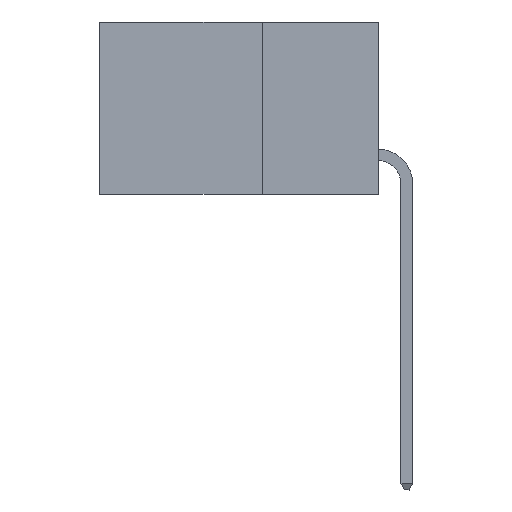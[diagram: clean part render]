
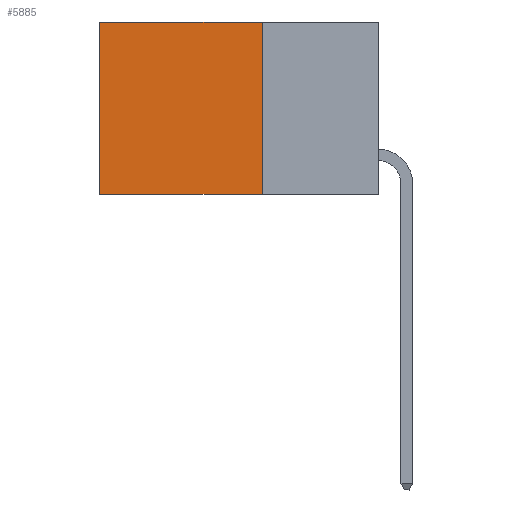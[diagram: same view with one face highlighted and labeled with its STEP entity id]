
A CAD part, left-side view. The second image highlights one B-rep face of the part: STEP entity #5885.
In plain terms, the highlighted planar face has unit normal (-1, 0, 0).
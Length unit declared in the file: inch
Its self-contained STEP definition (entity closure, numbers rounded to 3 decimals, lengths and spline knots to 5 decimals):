
#154 = EDGE_CURVE ( 'NONE', #14448, #2930, #10044, .T. ) ;
#266 = PLANE ( 'NONE',  #12601 ) ;
#954 = ORIENTED_EDGE ( 'NONE', *, *, #2855, .T. ) ;
#955 = CARTESIAN_POINT ( 'NONE',  ( 0.2615, 0.6, -0.37 ) ) ;
#1725 = ORIENTED_EDGE ( 'NONE', *, *, #154, .F. ) ;
#2405 = ORIENTED_EDGE ( 'NONE', *, *, #7330, .T. ) ;
#2855 = EDGE_CURVE ( 'NONE', #3892, #14859, #12479, .T. ) ;
#2923 = LINE ( 'NONE', #6515, #12404 ) ;
#2930 = VERTEX_POINT ( 'NONE', #11233 ) ;
#3892 = VERTEX_POINT ( 'NONE', #11964 ) ;
#5016 = DIRECTION ( 'NONE',  ( 0., 0., -1. ) ) ;
#5317 = CARTESIAN_POINT ( 'NONE',  ( 0.2615, 0.25, 0. ) ) ;
#5709 = DIRECTION ( 'NONE',  ( 0., 0., -1. ) ) ;
#5885 = ADVANCED_FACE ( 'NONE', ( #6194 ), #266, .F. ) ;
#6194 = FACE_OUTER_BOUND ( 'NONE', #13691, .T. ) ;
#6474 = CARTESIAN_POINT ( 'NONE',  ( 0.2615, 0.25, -0.37 ) ) ;
#6515 = CARTESIAN_POINT ( 'NONE',  ( 0.2615, 0.25, -0.37 ) ) ;
#7194 = CARTESIAN_POINT ( 'NONE',  ( 0.2615, 0.25, -0.37 ) ) ;
#7330 = EDGE_CURVE ( 'NONE', #14859, #2930, #11626, .T. ) ;
#8053 = EDGE_CURVE ( 'NONE', #3892, #14448, #2923, .T. ) ;
#8152 = VECTOR ( 'NONE', #5709, 39.37008 ) ;
#8535 = VECTOR ( 'NONE', #9901, 39.37008 ) ;
#9164 = DIRECTION ( 'NONE',  ( 0., 0., -1. ) ) ;
#9699 = CARTESIAN_POINT ( 'NONE',  ( 0.2615, 0.25, -0.37 ) ) ;
#9876 = CARTESIAN_POINT ( 'NONE',  ( 0.2615, 0.6, 0. ) ) ;
#9901 = DIRECTION ( 'NONE',  ( 0., 1., 0. ) ) ;
#10044 = LINE ( 'NONE', #6474, #8535 ) ;
#10938 = DIRECTION ( 'NONE',  ( 1., 0., 0. ) ) ;
#11233 = CARTESIAN_POINT ( 'NONE',  ( 0.2615, 0.6, -0.37 ) ) ;
#11626 = LINE ( 'NONE', #955, #8152 ) ;
#11964 = CARTESIAN_POINT ( 'NONE',  ( 0.2615, 0.25, 0. ) ) ;
#12078 = VECTOR ( 'NONE', #13729, 39.37008 ) ;
#12404 = VECTOR ( 'NONE', #9164, 39.37008 ) ;
#12479 = LINE ( 'NONE', #5317, #12078 ) ;
#12601 = AXIS2_PLACEMENT_3D ( 'NONE', #9699, #10938, #5016 ) ;
#13492 = ORIENTED_EDGE ( 'NONE', *, *, #8053, .F. ) ;
#13691 = EDGE_LOOP ( 'NONE', ( #2405, #1725, #13492, #954 ) ) ;
#13729 = DIRECTION ( 'NONE',  ( 0., 1., 0. ) ) ;
#14448 = VERTEX_POINT ( 'NONE', #7194 ) ;
#14859 = VERTEX_POINT ( 'NONE', #9876 ) ;
